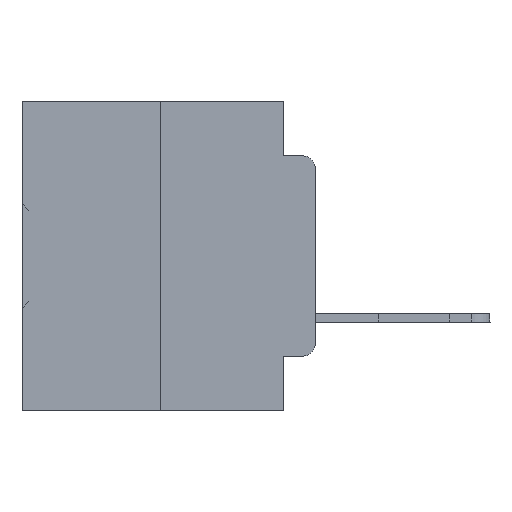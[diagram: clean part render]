
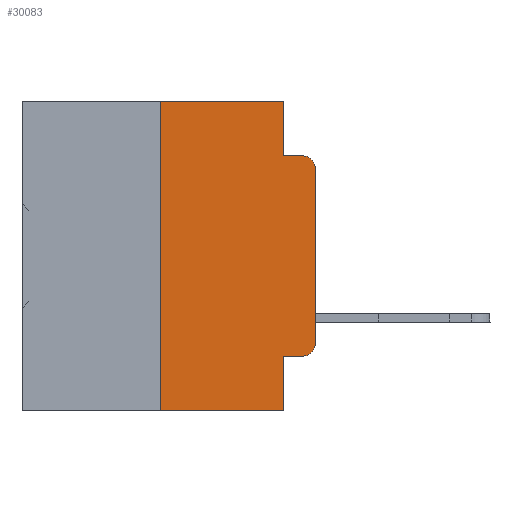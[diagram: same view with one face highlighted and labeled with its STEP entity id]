
A CAD part, left-side view. The second image highlights one B-rep face of the part: STEP entity #30083.
In plain terms, the highlighted planar face has unit normal (-1, 0, 0).
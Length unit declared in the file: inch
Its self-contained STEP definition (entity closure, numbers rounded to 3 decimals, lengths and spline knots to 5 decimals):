
#740 = CARTESIAN_POINT ( 'NONE',  ( 0., 0.473, 0. ) ) ;
#895 = VECTOR ( 'NONE', #12773, 39.37008 ) ;
#1078 = LINE ( 'NONE', #26597, #30333 ) ;
#1393 = CARTESIAN_POINT ( 'NONE',  ( 0., 0.02, -0.1085 ) ) ;
#1475 = LINE ( 'NONE', #12275, #13851 ) ;
#1671 = DIRECTION ( 'NONE',  ( 0., 0., 1. ) ) ;
#2664 = EDGE_CURVE ( 'NONE', #24916, #10504, #14836, .T. ) ;
#2818 = EDGE_CURVE ( 'NONE', #14945, #4499, #11294, .T. ) ;
#3152 = AXIS2_PLACEMENT_3D ( 'NONE', #740, #28827, #20197 ) ;
#3283 = DIRECTION ( 'NONE',  ( 0., -1., 0. ) ) ;
#3554 = VERTEX_POINT ( 'NONE', #4963 ) ;
#3724 = PLANE ( 'NONE',  #3152 ) ;
#4092 = LINE ( 'NONE', #6735, #33399 ) ;
#4499 = VERTEX_POINT ( 'NONE', #21425 ) ;
#4963 = CARTESIAN_POINT ( 'NONE',  ( 0., 0., -0.1085 ) ) ;
#6735 = CARTESIAN_POINT ( 'NONE',  ( 0., 0.473, 0. ) ) ;
#7489 = VERTEX_POINT ( 'NONE', #33629 ) ;
#7834 = CARTESIAN_POINT ( 'NONE',  ( 0., 0.051, -0.0885 ) ) ;
#8009 = ORIENTED_EDGE ( 'NONE', *, *, #8793, .T. ) ;
#8306 = ORIENTED_EDGE ( 'NONE', *, *, #25168, .F. ) ;
#8793 = EDGE_CURVE ( 'NONE', #24916, #21946, #16294, .T. ) ;
#8829 = EDGE_LOOP ( 'NONE', ( #15427, #16305, #30371, #8306, #34544, #31361, #8009, #18353, #11705, #36577 ) ) ;
#8919 = AXIS2_PLACEMENT_3D ( 'NONE', #1393, #15370, #12368 ) ;
#9069 = CARTESIAN_POINT ( 'NONE',  ( 0., 0.051, -0.5 ) ) ;
#10062 = AXIS2_PLACEMENT_3D ( 'NONE', #24515, #24634, #27079 ) ;
#10504 = VERTEX_POINT ( 'NONE', #19462 ) ;
#11108 = VECTOR ( 'NONE', #29027, 39.37008 ) ;
#11294 = CIRCLE ( 'NONE', #10062, 0.02 ) ;
#11705 = ORIENTED_EDGE ( 'NONE', *, *, #13372, .T. ) ;
#12275 = CARTESIAN_POINT ( 'NONE',  ( 0., 0.051, 0. ) ) ;
#12368 = DIRECTION ( 'NONE',  ( 0., 0., -1. ) ) ;
#12691 = CARTESIAN_POINT ( 'NONE',  ( 0., 0.02, -0.4115 ) ) ;
#12773 = DIRECTION ( 'NONE',  ( 0., 0., -1. ) ) ;
#13372 = EDGE_CURVE ( 'NONE', #7489, #14945, #22166, .T. ) ;
#13851 = VECTOR ( 'NONE', #15409, 39.37008 ) ;
#14318 = CIRCLE ( 'NONE', #8919, 0.02 ) ;
#14836 = LINE ( 'NONE', #15511, #25916 ) ;
#14877 = VERTEX_POINT ( 'NONE', #7834 ) ;
#14945 = VERTEX_POINT ( 'NONE', #12691 ) ;
#15370 = DIRECTION ( 'NONE',  ( -1., 0., 0. ) ) ;
#15409 = DIRECTION ( 'NONE',  ( 0., 0., -1. ) ) ;
#15427 = ORIENTED_EDGE ( 'NONE', *, *, #17822, .T. ) ;
#15511 = CARTESIAN_POINT ( 'NONE',  ( 0., 0.25, 0. ) ) ;
#16294 = LINE ( 'NONE', #17283, #27358 ) ;
#16305 = ORIENTED_EDGE ( 'NONE', *, *, #35694, .T. ) ;
#17283 = CARTESIAN_POINT ( 'NONE',  ( 0., 0.473, -0.5 ) ) ;
#17822 = EDGE_CURVE ( 'NONE', #4499, #3554, #19137, .T. ) ;
#18353 = ORIENTED_EDGE ( 'NONE', *, *, #32090, .F. ) ;
#18995 = CARTESIAN_POINT ( 'NONE',  ( 0., 0.02, -0.0885 ) ) ;
#19119 = EDGE_CURVE ( 'NONE', #14877, #26231, #1078, .T. ) ;
#19137 = LINE ( 'NONE', #26187, #11108 ) ;
#19462 = CARTESIAN_POINT ( 'NONE',  ( 0., 0.25, 0. ) ) ;
#20152 = EDGE_CURVE ( 'NONE', #10504, #29477, #4092, .T. ) ;
#20197 = DIRECTION ( 'NONE',  ( 0., 0., -1. ) ) ;
#20878 = DIRECTION ( 'NONE',  ( 0., -1., 0. ) ) ;
#21425 = CARTESIAN_POINT ( 'NONE',  ( 0., 0., -0.3915 ) ) ;
#21946 = VERTEX_POINT ( 'NONE', #9069 ) ;
#22166 = LINE ( 'NONE', #30292, #25649 ) ;
#23492 = LINE ( 'NONE', #29328, #895 ) ;
#24515 = CARTESIAN_POINT ( 'NONE',  ( 0., 0.02, -0.3915 ) ) ;
#24634 = DIRECTION ( 'NONE',  ( -1., 0., 0. ) ) ;
#24916 = VERTEX_POINT ( 'NONE', #26893 ) ;
#25168 = EDGE_CURVE ( 'NONE', #29477, #14877, #1475, .T. ) ;
#25649 = VECTOR ( 'NONE', #33064, 39.37008 ) ;
#25916 = VECTOR ( 'NONE', #1671, 39.37008 ) ;
#26187 = CARTESIAN_POINT ( 'NONE',  ( 0., 0., 0. ) ) ;
#26231 = VERTEX_POINT ( 'NONE', #18995 ) ;
#26597 = CARTESIAN_POINT ( 'NONE',  ( 0., 0.051, -0.0885 ) ) ;
#26893 = CARTESIAN_POINT ( 'NONE',  ( 0., 0.25, -0.5 ) ) ;
#27079 = DIRECTION ( 'NONE',  ( 0., 0., -1. ) ) ;
#27358 = VECTOR ( 'NONE', #3283, 39.37008 ) ;
#28827 = DIRECTION ( 'NONE',  ( 1., 0., 0. ) ) ;
#29027 = DIRECTION ( 'NONE',  ( 0., 0., 1. ) ) ;
#29328 = CARTESIAN_POINT ( 'NONE',  ( 0., 0.051, 0. ) ) ;
#29477 = VERTEX_POINT ( 'NONE', #34553 ) ;
#30083 = ADVANCED_FACE ( 'NONE', ( #36550 ), #3724, .F. ) ;
#30292 = CARTESIAN_POINT ( 'NONE',  ( 0., 0.051, -0.4115 ) ) ;
#30333 = VECTOR ( 'NONE', #32347, 39.37008 ) ;
#30371 = ORIENTED_EDGE ( 'NONE', *, *, #19119, .F. ) ;
#31361 = ORIENTED_EDGE ( 'NONE', *, *, #2664, .F. ) ;
#32090 = EDGE_CURVE ( 'NONE', #7489, #21946, #23492, .T. ) ;
#32347 = DIRECTION ( 'NONE',  ( 0., -1., 0. ) ) ;
#33064 = DIRECTION ( 'NONE',  ( 0., -1., 0. ) ) ;
#33399 = VECTOR ( 'NONE', #20878, 39.37008 ) ;
#33629 = CARTESIAN_POINT ( 'NONE',  ( 0., 0.051, -0.4115 ) ) ;
#34544 = ORIENTED_EDGE ( 'NONE', *, *, #20152, .F. ) ;
#34553 = CARTESIAN_POINT ( 'NONE',  ( 0., 0.051, 0. ) ) ;
#35694 = EDGE_CURVE ( 'NONE', #3554, #26231, #14318, .T. ) ;
#36550 = FACE_OUTER_BOUND ( 'NONE', #8829, .T. ) ;
#36577 = ORIENTED_EDGE ( 'NONE', *, *, #2818, .T. ) ;
